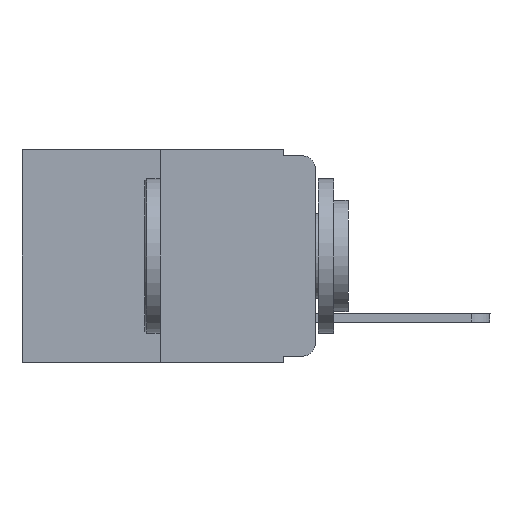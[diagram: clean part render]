
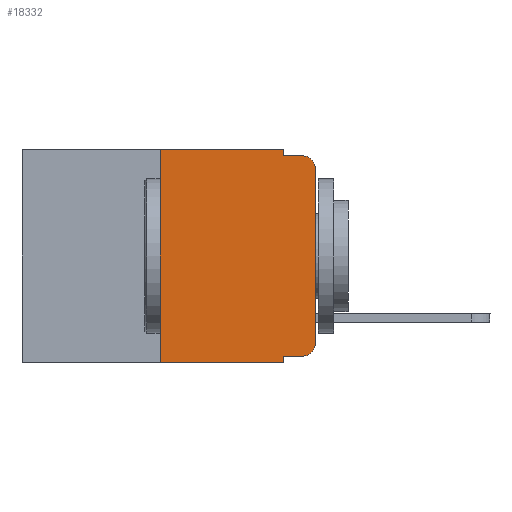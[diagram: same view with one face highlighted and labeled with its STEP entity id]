
A CAD part, left-side view. The second image highlights one B-rep face of the part: STEP entity #18332.
In plain terms, the highlighted planar face has unit normal (-1, 0, 0).
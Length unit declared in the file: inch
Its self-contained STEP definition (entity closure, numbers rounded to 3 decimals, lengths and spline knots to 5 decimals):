
#31 = CARTESIAN_POINT ( 'NONE',  ( 0., 0.051, 0. ) ) ;
#316 = CARTESIAN_POINT ( 'NONE',  ( 0., 0., -0.03 ) ) ;
#534 = DIRECTION ( 'NONE',  ( 0., -1., 0. ) ) ;
#716 = DIRECTION ( 'NONE',  ( 1., 0., 0. ) ) ;
#841 = CARTESIAN_POINT ( 'NONE',  ( 0., 0.473, -0.343 ) ) ;
#1064 = CARTESIAN_POINT ( 'NONE',  ( 0., 0.02, -0.01 ) ) ;
#1076 = LINE ( 'NONE', #20844, #14591 ) ;
#1376 = LINE ( 'NONE', #841, #17856 ) ;
#1440 = VECTOR ( 'NONE', #11400, 39.37008 ) ;
#1858 = VERTEX_POINT ( 'NONE', #9205 ) ;
#1871 = CARTESIAN_POINT ( 'NONE',  ( 0., 0., -0.313 ) ) ;
#2092 = EDGE_CURVE ( 'NONE', #14833, #12349, #1376, .T. ) ;
#2959 = DIRECTION ( 'NONE',  ( 0., 0., 1. ) ) ;
#3292 = CARTESIAN_POINT ( 'NONE',  ( 0., 0.051, -0.01 ) ) ;
#3751 = EDGE_CURVE ( 'NONE', #18809, #12349, #19647, .T. ) ;
#4155 = VECTOR ( 'NONE', #14720, 39.37008 ) ;
#4517 = DIRECTION ( 'NONE',  ( 0., 0., -1. ) ) ;
#5122 = VECTOR ( 'NONE', #12142, 39.37008 ) ;
#6663 = EDGE_CURVE ( 'NONE', #1858, #16939, #8741, .T. ) ;
#6911 = VECTOR ( 'NONE', #2959, 39.37008 ) ;
#7499 = DIRECTION ( 'NONE',  ( 0., 0., -1. ) ) ;
#7581 = PLANE ( 'NONE',  #16314 ) ;
#7749 = CARTESIAN_POINT ( 'NONE',  ( 0., 0.473, 0. ) ) ;
#7769 = LINE ( 'NONE', #31, #11833 ) ;
#7989 = CARTESIAN_POINT ( 'NONE',  ( 0., 0.02, -0.313 ) ) ;
#8741 = LINE ( 'NONE', #7749, #4155 ) ;
#8758 = ORIENTED_EDGE ( 'NONE', *, *, #2092, .T. ) ;
#8826 = EDGE_LOOP ( 'NONE', ( #11586, #14977, #9508, #15927, #8857, #14036, #8758, #11128, #13007, #14723 ) ) ;
#8857 = ORIENTED_EDGE ( 'NONE', *, *, #6663, .F. ) ;
#8877 = EDGE_CURVE ( 'NONE', #21774, #10618, #19182, .T. ) ;
#9205 = CARTESIAN_POINT ( 'NONE',  ( 0., 0.25, 0. ) ) ;
#9401 = CARTESIAN_POINT ( 'NONE',  ( 0., 0.02, -0.333 ) ) ;
#9508 = ORIENTED_EDGE ( 'NONE', *, *, #8877, .F. ) ;
#10199 = CARTESIAN_POINT ( 'NONE',  ( 0., 0.051, 0. ) ) ;
#10618 = VERTEX_POINT ( 'NONE', #1064 ) ;
#10978 = EDGE_CURVE ( 'NONE', #14833, #1858, #19362, .T. ) ;
#11128 = ORIENTED_EDGE ( 'NONE', *, *, #3751, .F. ) ;
#11291 = DIRECTION ( 'NONE',  ( -1., 0., 0. ) ) ;
#11400 = DIRECTION ( 'NONE',  ( 0., 0., 1. ) ) ;
#11586 = ORIENTED_EDGE ( 'NONE', *, *, #13049, .T. ) ;
#11592 = EDGE_CURVE ( 'NONE', #14109, #20177, #13381, .T. ) ;
#11833 = VECTOR ( 'NONE', #15531, 39.37008 ) ;
#11955 = LINE ( 'NONE', #13228, #1440 ) ;
#12142 = DIRECTION ( 'NONE',  ( 0., -1., 0. ) ) ;
#12349 = VERTEX_POINT ( 'NONE', #16067 ) ;
#13007 = ORIENTED_EDGE ( 'NONE', *, *, #15926, .T. ) ;
#13049 = EDGE_CURVE ( 'NONE', #20177, #17193, #11955, .T. ) ;
#13080 = CARTESIAN_POINT ( 'NONE',  ( 0., 0.25, -0.343 ) ) ;
#13228 = CARTESIAN_POINT ( 'NONE',  ( 0., 0., 0. ) ) ;
#13381 = CIRCLE ( 'NONE', #17231, 0.02 ) ;
#13753 = DIRECTION ( 'NONE',  ( 0., -1., 0. ) ) ;
#14036 = ORIENTED_EDGE ( 'NONE', *, *, #10978, .F. ) ;
#14109 = VERTEX_POINT ( 'NONE', #9401 ) ;
#14591 = VECTOR ( 'NONE', #13753, 39.37008 ) ;
#14720 = DIRECTION ( 'NONE',  ( 0., -1., 0. ) ) ;
#14723 = ORIENTED_EDGE ( 'NONE', *, *, #11592, .T. ) ;
#14776 = CIRCLE ( 'NONE', #17745, 0.02 ) ;
#14833 = VERTEX_POINT ( 'NONE', #13080 ) ;
#14977 = ORIENTED_EDGE ( 'NONE', *, *, #17864, .T. ) ;
#15531 = DIRECTION ( 'NONE',  ( 0., 0., -1. ) ) ;
#15926 = EDGE_CURVE ( 'NONE', #18809, #14109, #1076, .T. ) ;
#15927 = ORIENTED_EDGE ( 'NONE', *, *, #17022, .F. ) ;
#16067 = CARTESIAN_POINT ( 'NONE',  ( 0., 0.051, -0.343 ) ) ;
#16314 = AXIS2_PLACEMENT_3D ( 'NONE', #19462, #716, #7499 ) ;
#16908 = CARTESIAN_POINT ( 'NONE',  ( 0., 0.051, -0.01 ) ) ;
#16939 = VERTEX_POINT ( 'NONE', #10199 ) ;
#17022 = EDGE_CURVE ( 'NONE', #16939, #21774, #7769, .T. ) ;
#17144 = CARTESIAN_POINT ( 'NONE',  ( 0., 0.051, -0.333 ) ) ;
#17193 = VERTEX_POINT ( 'NONE', #316 ) ;
#17217 = FACE_OUTER_BOUND ( 'NONE', #8826, .T. ) ;
#17231 = AXIS2_PLACEMENT_3D ( 'NONE', #7989, #21829, #22281 ) ;
#17745 = AXIS2_PLACEMENT_3D ( 'NONE', #21577, #11291, #4517 ) ;
#17856 = VECTOR ( 'NONE', #534, 39.37008 ) ;
#17864 = EDGE_CURVE ( 'NONE', #17193, #10618, #14776, .T. ) ;
#17987 = CARTESIAN_POINT ( 'NONE',  ( 0., 0.25, 0. ) ) ;
#18332 = ADVANCED_FACE ( 'NONE', ( #17217 ), #7581, .F. ) ;
#18591 = VECTOR ( 'NONE', #21618, 39.37008 ) ;
#18809 = VERTEX_POINT ( 'NONE', #17144 ) ;
#19182 = LINE ( 'NONE', #3292, #5122 ) ;
#19362 = LINE ( 'NONE', #17987, #6911 ) ;
#19462 = CARTESIAN_POINT ( 'NONE',  ( 0., 0.473, 0. ) ) ;
#19647 = LINE ( 'NONE', #20126, #18591 ) ;
#20126 = CARTESIAN_POINT ( 'NONE',  ( 0., 0.051, 0. ) ) ;
#20177 = VERTEX_POINT ( 'NONE', #1871 ) ;
#20844 = CARTESIAN_POINT ( 'NONE',  ( 0., 0.051, -0.333 ) ) ;
#21577 = CARTESIAN_POINT ( 'NONE',  ( 0., 0.02, -0.03 ) ) ;
#21618 = DIRECTION ( 'NONE',  ( 0., 0., -1. ) ) ;
#21774 = VERTEX_POINT ( 'NONE', #16908 ) ;
#21829 = DIRECTION ( 'NONE',  ( -1., 0., 0. ) ) ;
#22281 = DIRECTION ( 'NONE',  ( 0., 0., -1. ) ) ;
